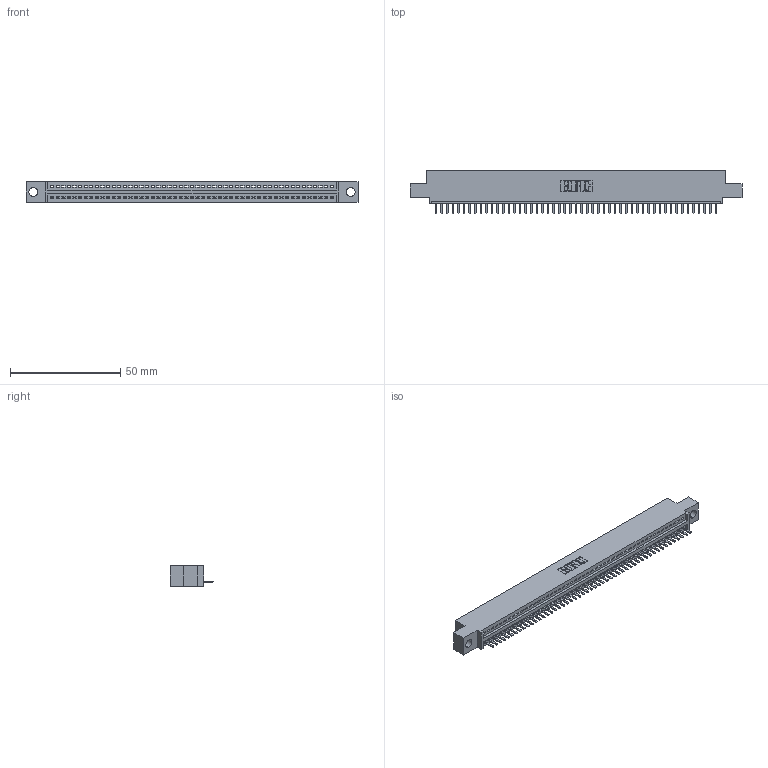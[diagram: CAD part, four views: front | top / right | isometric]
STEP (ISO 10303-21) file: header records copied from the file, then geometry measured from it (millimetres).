
FILE_DESCRIPTION (( 'STEP AP203' ), '1' );
FILE_NAME ('345-051-520-404.STEP', '2021-05-28T15:23:08', ( '' ), ( '' ), 'SwSTEP 2.0', 'SolidWorks 2020', '' );
FILE_SCHEMA (( 'CONFIG_CONTROL_DESIGN' ));
Length unit declared in the file: inch
Products named in the file (3): 345 Part_0.110 Offset - 0.156 Dia-TI; 345-292-001_345-293-120; 345-051-520-404
Assembly tree (52 placements, depth 2):
  345-051-520-404
    345 Part_0.110 Offset - 0.156 Dia-TI
    345-292-001_345-293-120  x51
Bounding box: 150.75 x 19.68 x 9.4 mm (x, y, z)
Volume: 14066 mm3; surface area: 18259.2 mm2
Topology: 52 solids, 52 shells, 3306 faces, 9773 edges, 6378 vertices
Faces by surface type: plane 2240, cylinder 1066
Entity records: 37837 total; most frequent: CARTESIAN_POINT 6575, ORIENTED_EDGE 6546, DIRECTION 5715, EDGE_CURVE 3273, VECTOR 2933, LINE 2933, VERTEX_POINT 2178, AXIS2_PLACEMENT_3D 1391
